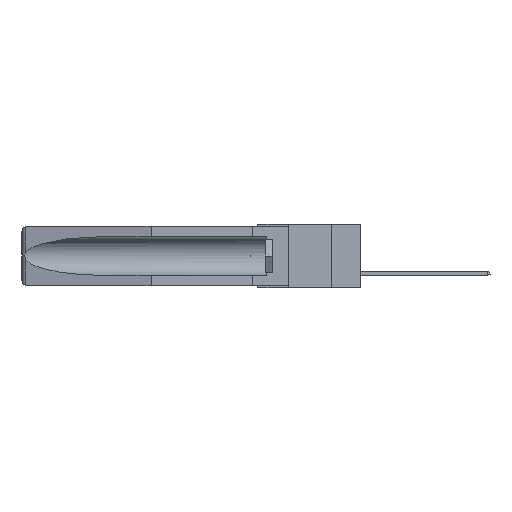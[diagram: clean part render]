
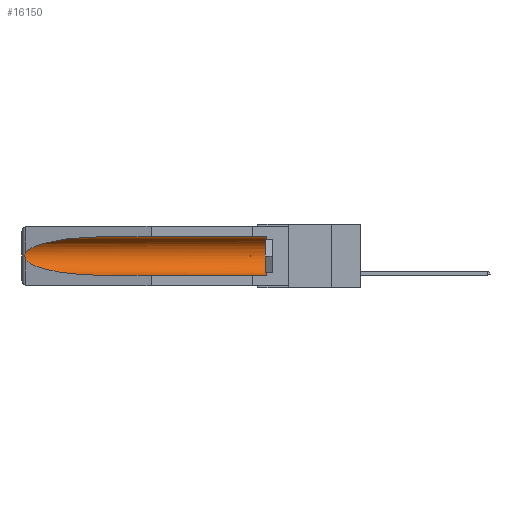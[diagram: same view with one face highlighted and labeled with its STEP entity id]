
A CAD part, left-side view. The second image highlights one B-rep face of the part: STEP entity #16150.
In plain terms, the highlighted cylindrical face has radius 2.857 mm (diameter 5.715 mm), a partial arc.
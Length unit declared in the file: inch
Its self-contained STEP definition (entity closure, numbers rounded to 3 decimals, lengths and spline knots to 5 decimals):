
#497 = CARTESIAN_POINT ( 'NONE',  ( 0.155, 1.07973, -0.059 ) ) ;
#632 = DIRECTION ( 'NONE',  ( 0., -1., 0. ) ) ;
#802 = VECTOR ( 'NONE', #24856, 39.37008 ) ;
#1410 = CARTESIAN_POINT ( 'NONE',  ( 0.26537, 1.52718, -0.14972 ) ) ;
#1508 = VERTEX_POINT ( 'NONE', #15337 ) ;
#1528 = CARTESIAN_POINT ( 'NONE',  ( 0.26537, 1.52718, -0.19328 ) ) ;
#1530 = FACE_OUTER_BOUND ( 'NONE', #32174, .T. ) ;
#1945 = CARTESIAN_POINT ( 'NONE',  ( 0.155, -0.30754, -0.284 ) ) ;
#2347 = CARTESIAN_POINT ( 'NONE',  ( 0.155, 1.07973, -0.284 ) ) ;
#3456 = CARTESIAN_POINT ( 'NONE',  ( 0.21114, 1.30732, -0.059 ) ) ;
#3802 = VERTEX_POINT ( 'NONE', #17394 ) ;
#3873 = CARTESIAN_POINT ( 'NONE',  ( 0.155, 0.126, -0.059 ) ) ;
#4033 = CARTESIAN_POINT ( 'NONE',  ( 0.2675, 1.53308, -0.16763 ) ) ;
#7791 = CARTESIAN_POINT ( 'NONE',  ( 0.155, -0.30754, -0.059 ) ) ;
#7869 = AXIS2_PLACEMENT_3D ( 'NONE', #8627, #16504, #24473 ) ;
#8262 = ORIENTED_EDGE ( 'NONE', *, *, #23599, .T. ) ;
#8436 = DIRECTION ( 'NONE',  ( 0., 0., 1. ) ) ;
#8596 = CARTESIAN_POINT ( 'NONE',  ( 0.21114, 1.30732, -0.284 ) ) ;
#8627 = CARTESIAN_POINT ( 'NONE',  ( 0.155, -0.30754, -0.1715 ) ) ;
#8752 = CARTESIAN_POINT ( 'NONE',  ( 0.25451, 1.48313, -0.09465 ) ) ;
#9102 = CARTESIAN_POINT ( 'NONE',  ( 0.2675, 1.53308, -0.17534 ) ) ;
#9916 = VERTEX_POINT ( 'NONE', #3873 ) ;
#10479 =( BOUNDED_CURVE ( )  B_SPLINE_CURVE ( 3, ( #24220, #27066, #8596, #26830 ),
 .UNSPECIFIED., .F., .F. ) 
 B_SPLINE_CURVE_WITH_KNOTS ( ( 4, 4 ),
 ( 0.1948, 1.5708 ),
 .UNSPECIFIED. ) 
 CURVE ( )  GEOMETRIC_REPRESENTATION_ITEM ( )  RATIONAL_B_SPLINE_CURVE ( ( 1., 0.848, 0.848, 1. ) ) 
 REPRESENTATION_ITEM ( '' )  );
#10723 = EDGE_CURVE ( 'NONE', #21154, #22412, #13929, .T. ) ;
#11284 = CARTESIAN_POINT ( 'NONE',  ( 0.26537, 1.52718, -0.14972 ) ) ;
#13116 = VECTOR ( 'NONE', #28678, 39.37008 ) ;
#13819 = ORIENTED_EDGE ( 'NONE', *, *, #22513, .T. ) ;
#13929 = LINE ( 'NONE', #1945, #802 ) ;
#14252 = CARTESIAN_POINT ( 'NONE',  ( 0.26654, 1.53092, -0.15636 ) ) ;
#14638 = B_SPLINE_CURVE_WITH_KNOTS ( 'NONE', 3,
 ( #1410, #19827, #14252, #17097, #4033, #9102, #16982, #16878, #17209, #1528 ),
 .UNSPECIFIED., .F., .F.,
 ( 4, 2, 2, 2, 4 ),
 ( 0., 0.00029, 0.00058, 0.00087, 0.00117 ),
 .UNSPECIFIED. ) ;
#15337 = CARTESIAN_POINT ( 'NONE',  ( 0.155, 1.07973, -0.059 ) ) ;
#15907 = CIRCLE ( 'NONE', #18573, 0.1125 ) ;
#16150 = ADVANCED_FACE ( 'NONE', ( #1530 ), #29769, .F. ) ;
#16504 = DIRECTION ( 'NONE',  ( 0., 1., 0. ) ) ;
#16735 = CARTESIAN_POINT ( 'NONE',  ( 0.155, 0.126, -0.284 ) ) ;
#16878 = CARTESIAN_POINT ( 'NONE',  ( 0.26655, 1.53094, -0.18657 ) ) ;
#16982 = CARTESIAN_POINT ( 'NONE',  ( 0.2673, 1.53269, -0.17917 ) ) ;
#17097 = CARTESIAN_POINT ( 'NONE',  ( 0.2673, 1.5327, -0.16383 ) ) ;
#17209 = CARTESIAN_POINT ( 'NONE',  ( 0.26597, 1.5296, -0.19026 ) ) ;
#17385 =( BOUNDED_CURVE ( )  B_SPLINE_CURVE ( 3, ( #497, #3456, #8752, #18805 ),
 .UNSPECIFIED., .F., .F. ) 
 B_SPLINE_CURVE_WITH_KNOTS ( ( 4, 4 ),
 ( 4.71239, 6.08839 ),
 .UNSPECIFIED. ) 
 CURVE ( )  GEOMETRIC_REPRESENTATION_ITEM ( )  RATIONAL_B_SPLINE_CURVE ( ( 1., 0.848, 0.848, 1. ) ) 
 REPRESENTATION_ITEM ( '' )  );
#17394 = CARTESIAN_POINT ( 'NONE',  ( 0.26537, 1.52718, -0.19328 ) ) ;
#18573 = AXIS2_PLACEMENT_3D ( 'NONE', #21128, #632, #8436 ) ;
#18746 = EDGE_CURVE ( 'NONE', #1508, #25861, #17385, .T. ) ;
#18805 = CARTESIAN_POINT ( 'NONE',  ( 0.26537, 1.52718, -0.14972 ) ) ;
#18957 = ORIENTED_EDGE ( 'NONE', *, *, #29050, .T. ) ;
#19424 = ORIENTED_EDGE ( 'NONE', *, *, #10723, .F. ) ;
#19827 = CARTESIAN_POINT ( 'NONE',  ( 0.26597, 1.52961, -0.15275 ) ) ;
#20272 = ORIENTED_EDGE ( 'NONE', *, *, #18746, .T. ) ;
#20465 = EDGE_CURVE ( 'NONE', #9916, #1508, #29040, .T. ) ;
#21128 = CARTESIAN_POINT ( 'NONE',  ( 0.155, 0.126, -0.1715 ) ) ;
#21154 = VERTEX_POINT ( 'NONE', #16735 ) ;
#22412 = VERTEX_POINT ( 'NONE', #2347 ) ;
#22513 = EDGE_CURVE ( 'NONE', #21154, #9916, #15907, .T. ) ;
#23599 = EDGE_CURVE ( 'NONE', #3802, #22412, #10479, .T. ) ;
#24220 = CARTESIAN_POINT ( 'NONE',  ( 0.26537, 1.52718, -0.19328 ) ) ;
#24473 = DIRECTION ( 'NONE',  ( 0., 0., 1. ) ) ;
#24856 = DIRECTION ( 'NONE',  ( 0., 1., 0. ) ) ;
#25861 = VERTEX_POINT ( 'NONE', #11284 ) ;
#26817 = ORIENTED_EDGE ( 'NONE', *, *, #20465, .T. ) ;
#26830 = CARTESIAN_POINT ( 'NONE',  ( 0.155, 1.07973, -0.284 ) ) ;
#27066 = CARTESIAN_POINT ( 'NONE',  ( 0.25451, 1.48313, -0.24835 ) ) ;
#28678 = DIRECTION ( 'NONE',  ( 0., 1., 0. ) ) ;
#29040 = LINE ( 'NONE', #7791, #13116 ) ;
#29050 = EDGE_CURVE ( 'NONE', #25861, #3802, #14638, .T. ) ;
#29769 = CYLINDRICAL_SURFACE ( 'NONE', #7869, 0.1125 ) ;
#32174 = EDGE_LOOP ( 'NONE', ( #20272, #18957, #8262, #19424, #13819, #26817 ) ) ;
